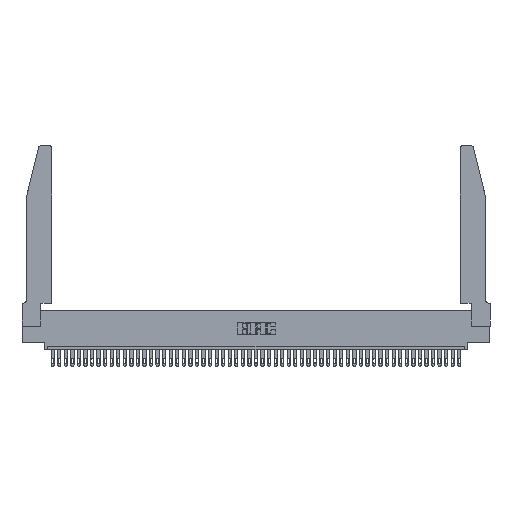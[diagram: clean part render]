
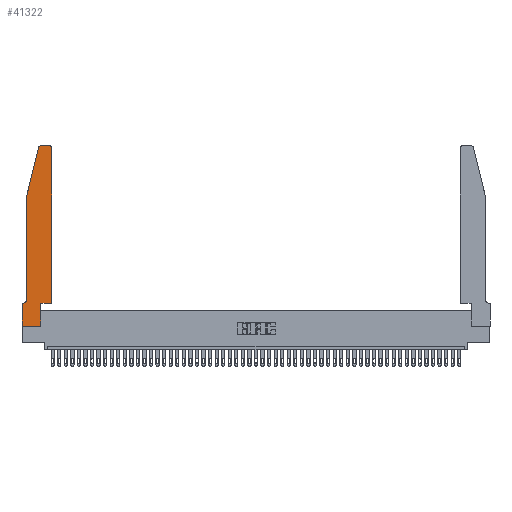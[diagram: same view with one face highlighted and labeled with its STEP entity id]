
A CAD part, top view. The second image highlights one B-rep face of the part: STEP entity #41322.
In plain terms, the highlighted planar face has unit normal (0, 0, 1).
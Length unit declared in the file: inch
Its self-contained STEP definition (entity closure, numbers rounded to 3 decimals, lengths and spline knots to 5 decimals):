
#293 = LINE ( 'NONE', #36253, #9232 ) ;
#1003 = CARTESIAN_POINT ( 'NONE',  ( 0.284, 2.75, 0.37 ) ) ;
#1127 = CIRCLE ( 'NONE', #5654, 0.03 ) ;
#1502 = CARTESIAN_POINT ( 'NONE',  ( 0.284, 2.72, 0.37 ) ) ;
#1766 = AXIS2_PLACEMENT_3D ( 'NONE', #15283, #30961, #38581 ) ;
#1912 = CARTESIAN_POINT ( 'NONE',  ( 0.4505, 0.35, 0.37 ) ) ;
#3113 = VECTOR ( 'NONE', #17878, 39.37008 ) ;
#3418 = VECTOR ( 'NONE', #46422, 39.37008 ) ;
#4166 = ORIENTED_EDGE ( 'NONE', *, *, #16617, .T. ) ;
#4878 = LINE ( 'NONE', #1912, #3113 ) ;
#5654 = AXIS2_PLACEMENT_3D ( 'NONE', #20424, #35620, #36146 ) ;
#5821 = DIRECTION ( 'NONE',  ( -1., 0., 0. ) ) ;
#5923 = DIRECTION ( 'NONE',  ( 1., 0., 0. ) ) ;
#6337 = ORIENTED_EDGE ( 'NONE', *, *, #7967, .T. ) ;
#6805 = ORIENTED_EDGE ( 'NONE', *, *, #33652, .T. ) ;
#7450 = ORIENTED_EDGE ( 'NONE', *, *, #42451, .T. ) ;
#7945 = AXIS2_PLACEMENT_3D ( 'NONE', #1502, #29019, #36858 ) ;
#7967 = EDGE_CURVE ( 'NONE', #21422, #33467, #32588, .T. ) ;
#8761 = CARTESIAN_POINT ( 'NONE',  ( 0., 0.35, 0.37 ) ) ;
#8895 = LINE ( 'NONE', #34844, #48985 ) ;
#9232 = VECTOR ( 'NONE', #12668, 39.37008 ) ;
#10984 = CARTESIAN_POINT ( 'NONE',  ( 0., 0., 0.37 ) ) ;
#11817 = VECTOR ( 'NONE', #30785, 39.37008 ) ;
#11987 = VECTOR ( 'NONE', #47247, 39.37008 ) ;
#12173 = CARTESIAN_POINT ( 'NONE',  ( 0.0755, 2., 0.37 ) ) ;
#12430 = PLANE ( 'NONE',  #16178 ) ;
#12448 = EDGE_CURVE ( 'NONE', #44866, #32060, #45692, .T. ) ;
#12668 = DIRECTION ( 'NONE',  ( 0., -1., 0. ) ) ;
#13068 = ORIENTED_EDGE ( 'NONE', *, *, #24376, .T. ) ;
#15273 = VERTEX_POINT ( 'NONE', #12173 ) ;
#15283 = CARTESIAN_POINT ( 'NONE',  ( 0.0055, 0.42, 0.37 ) ) ;
#16151 = LINE ( 'NONE', #35203, #11987 ) ;
#16178 = AXIS2_PLACEMENT_3D ( 'NONE', #8761, #35126, #19426 ) ;
#16309 = CARTESIAN_POINT ( 'NONE',  ( 0.4505, 0.35, 0.37 ) ) ;
#16617 = EDGE_CURVE ( 'NONE', #33467, #39582, #45801, .T. ) ;
#17650 = ORIENTED_EDGE ( 'NONE', *, *, #20066, .T. ) ;
#17878 = DIRECTION ( 'NONE',  ( 0., 1., 0. ) ) ;
#19426 = DIRECTION ( 'NONE',  ( 1., 0., 0. ) ) ;
#19821 = VERTEX_POINT ( 'NONE', #48786 ) ;
#19915 = DIRECTION ( 'NONE',  ( 1., 0., 0. ) ) ;
#20066 = EDGE_CURVE ( 'NONE', #47333, #19821, #4878, .T. ) ;
#20276 = VECTOR ( 'NONE', #19915, 39.37008 ) ;
#20424 = CARTESIAN_POINT ( 'NONE',  ( 0.4205, 2.72, 0.37 ) ) ;
#21422 = VERTEX_POINT ( 'NONE', #40353 ) ;
#21448 = LINE ( 'NONE', #22476, #11817 ) ;
#22006 = VERTEX_POINT ( 'NONE', #31861 ) ;
#22476 = CARTESIAN_POINT ( 'NONE',  ( 0., 0., 0.37 ) ) ;
#22952 = VECTOR ( 'NONE', #5821, 39.37008 ) ;
#23239 = CARTESIAN_POINT ( 'NONE',  ( 0.0055, 0.35, 0.37 ) ) ;
#24376 = EDGE_CURVE ( 'NONE', #41069, #25313, #43608, .T. ) ;
#25313 = VERTEX_POINT ( 'NONE', #39078 ) ;
#26601 = FACE_OUTER_BOUND ( 'NONE', #36232, .T. ) ;
#27374 = CARTESIAN_POINT ( 'NONE',  ( 0.4505, 0.35, 0.37 ) ) ;
#27750 = LINE ( 'NONE', #45148, #22952 ) ;
#28246 = LINE ( 'NONE', #27374, #45604 ) ;
#29019 = DIRECTION ( 'NONE',  ( 0., 0., 1. ) ) ;
#29709 = EDGE_CURVE ( 'NONE', #48784, #44866, #27750, .T. ) ;
#30178 = ORIENTED_EDGE ( 'NONE', *, *, #33738, .T. ) ;
#30785 = DIRECTION ( 'NONE',  ( 0., -1., 0. ) ) ;
#30961 = DIRECTION ( 'NONE',  ( 0., 0., -1. ) ) ;
#31861 = CARTESIAN_POINT ( 'NONE',  ( 0.2865, 0.35, 0.37 ) ) ;
#31894 = CARTESIAN_POINT ( 'NONE',  ( 0.25487, 2.72718, 0.37 ) ) ;
#32060 = VERTEX_POINT ( 'NONE', #31894 ) ;
#32071 = EDGE_CURVE ( 'NONE', #32060, #15273, #16151, .T. ) ;
#32588 = CIRCLE ( 'NONE', #1766, 0.07 ) ;
#33406 = CARTESIAN_POINT ( 'NONE',  ( 0.4205, 2.75, 0.37 ) ) ;
#33467 = VERTEX_POINT ( 'NONE', #23239 ) ;
#33652 = EDGE_CURVE ( 'NONE', #39582, #41069, #21448, .T. ) ;
#33738 = EDGE_CURVE ( 'NONE', #19821, #48784, #1127, .T. ) ;
#34844 = CARTESIAN_POINT ( 'NONE',  ( 0.2865, 0.35, 0.37 ) ) ;
#35126 = DIRECTION ( 'NONE',  ( 0., 0., 1. ) ) ;
#35190 = DIRECTION ( 'NONE',  ( 0., 1., 0. ) ) ;
#35203 = CARTESIAN_POINT ( 'NONE',  ( 0.0755, 2., 0.37 ) ) ;
#35620 = DIRECTION ( 'NONE',  ( 0., 0., 1. ) ) ;
#36112 = ORIENTED_EDGE ( 'NONE', *, *, #29709, .T. ) ;
#36146 = DIRECTION ( 'NONE',  ( 1., 0., 0. ) ) ;
#36232 = EDGE_LOOP ( 'NONE', ( #36112, #38979, #37041, #42338, #6337, #4166, #6805, #13068, #36638, #7450, #17650, #30178 ) ) ;
#36253 = CARTESIAN_POINT ( 'NONE',  ( 0.0755, 2., 0.37 ) ) ;
#36638 = ORIENTED_EDGE ( 'NONE', *, *, #38869, .T. ) ;
#36858 = DIRECTION ( 'NONE',  ( 1., 0., 0. ) ) ;
#37041 = ORIENTED_EDGE ( 'NONE', *, *, #32071, .T. ) ;
#38558 = CARTESIAN_POINT ( 'NONE',  ( 0.0755, 0.35, 0.37 ) ) ;
#38581 = DIRECTION ( 'NONE',  ( -1., 0., 0. ) ) ;
#38869 = EDGE_CURVE ( 'NONE', #25313, #22006, #8895, .T. ) ;
#38979 = ORIENTED_EDGE ( 'NONE', *, *, #12448, .T. ) ;
#39078 = CARTESIAN_POINT ( 'NONE',  ( 0.2865, 0., 0.37 ) ) ;
#39582 = VERTEX_POINT ( 'NONE', #43352 ) ;
#40353 = CARTESIAN_POINT ( 'NONE',  ( 0.0755, 0.42, 0.37 ) ) ;
#41069 = VERTEX_POINT ( 'NONE', #10984 ) ;
#41322 = ADVANCED_FACE ( 'NONE', ( #26601 ), #12430, .T. ) ;
#41597 = EDGE_CURVE ( 'NONE', #15273, #21422, #293, .T. ) ;
#42338 = ORIENTED_EDGE ( 'NONE', *, *, #41597, .T. ) ;
#42451 = EDGE_CURVE ( 'NONE', #22006, #47333, #28246, .T. ) ;
#43352 = CARTESIAN_POINT ( 'NONE',  ( 0., 0.35, 0.37 ) ) ;
#43608 = LINE ( 'NONE', #43885, #20276 ) ;
#43885 = CARTESIAN_POINT ( 'NONE',  ( 0., 0., 0.37 ) ) ;
#44866 = VERTEX_POINT ( 'NONE', #1003 ) ;
#45148 = CARTESIAN_POINT ( 'NONE',  ( 0.2605, 2.75, 0.37 ) ) ;
#45604 = VECTOR ( 'NONE', #5923, 39.37008 ) ;
#45692 = CIRCLE ( 'NONE', #7945, 0.03 ) ;
#45801 = LINE ( 'NONE', #38558, #3418 ) ;
#46422 = DIRECTION ( 'NONE',  ( -1., 0., 0. ) ) ;
#47247 = DIRECTION ( 'NONE',  ( -0.239, -0.971, 0. ) ) ;
#47333 = VERTEX_POINT ( 'NONE', #16309 ) ;
#48784 = VERTEX_POINT ( 'NONE', #33406 ) ;
#48786 = CARTESIAN_POINT ( 'NONE',  ( 0.4505, 2.72, 0.37 ) ) ;
#48985 = VECTOR ( 'NONE', #35190, 39.37008 ) ;
